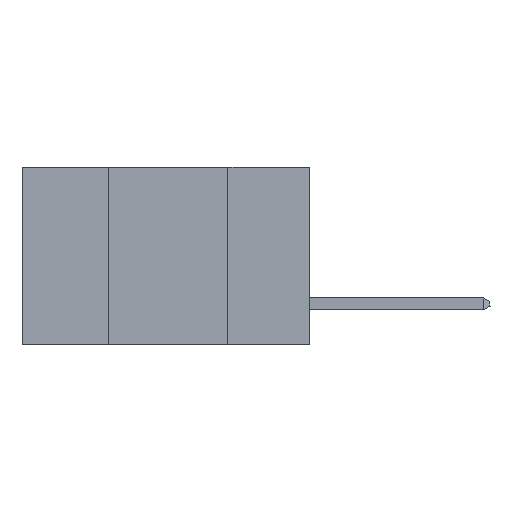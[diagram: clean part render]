
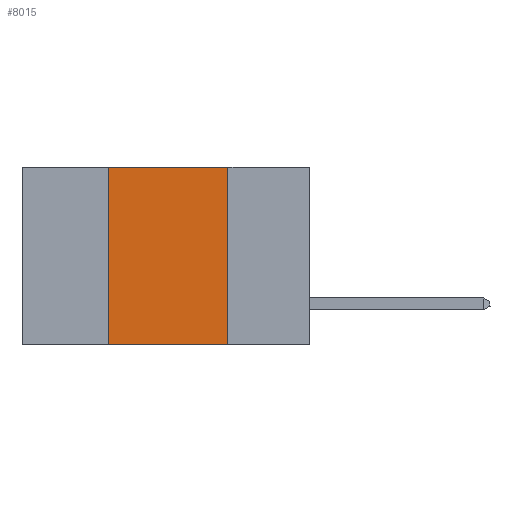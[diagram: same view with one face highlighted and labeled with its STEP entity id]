
A CAD part, left-side view. The second image highlights one B-rep face of the part: STEP entity #8015.
In plain terms, the highlighted planar face has unit normal (-1, 0, 0).
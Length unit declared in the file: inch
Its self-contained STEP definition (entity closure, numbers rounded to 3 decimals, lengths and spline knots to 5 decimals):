
#1480 = VERTEX_POINT ( 'NONE', #7869 ) ;
#1724 = ORIENTED_EDGE ( 'NONE', *, *, #2105, .F. ) ;
#2105 = EDGE_CURVE ( 'NONE', #18420, #6657, #20396, .T. ) ;
#2632 = VERTEX_POINT ( 'NONE', #9596 ) ;
#2825 = LINE ( 'NONE', #15860, #6782 ) ;
#4143 = EDGE_LOOP ( 'NONE', ( #13917, #4170, #1724, #4191 ) ) ;
#4170 = ORIENTED_EDGE ( 'NONE', *, *, #18962, .F. ) ;
#4191 = ORIENTED_EDGE ( 'NONE', *, *, #20231, .T. ) ;
#4377 = CARTESIAN_POINT ( 'NONE',  ( 0., 0.17, 0. ) ) ;
#4565 = VECTOR ( 'NONE', #16629, 39.37008 ) ;
#4564 = DIRECTION ( 'NONE',  ( 0., 0., -1. ) ) ;
#5582 = DIRECTION ( 'NONE',  ( 0., -1., 0. ) ) ;
#6474 = FACE_OUTER_BOUND ( 'NONE', #4143, .T. ) ;
#6653 = CARTESIAN_POINT ( 'NONE',  ( 0., 0.42, 0. ) ) ;
#6657 = VERTEX_POINT ( 'NONE', #16214 ) ;
#6782 = VECTOR ( 'NONE', #5582, 39.37008 ) ;
#7869 = CARTESIAN_POINT ( 'NONE',  ( 0., 0.17, 0. ) ) ;
#8015 = ADVANCED_FACE ( 'NONE', ( #6474 ), #12578, .F. ) ;
#9596 = CARTESIAN_POINT ( 'NONE',  ( 0., 0.17, -0.37 ) ) ;
#10068 = DIRECTION ( 'NONE',  ( 0., 0., -1. ) ) ;
#10157 = VECTOR ( 'NONE', #18342, 39.37008 ) ;
#10955 = CARTESIAN_POINT ( 'NONE',  ( 0., 0.6, 0. ) ) ;
#12189 = VECTOR ( 'NONE', #10068, 39.37008 ) ;
#12578 = PLANE ( 'NONE',  #15012 ) ;
#13059 = LINE ( 'NONE', #18613, #10157 ) ;
#13917 = ORIENTED_EDGE ( 'NONE', *, *, #21399, .F. ) ;
#14598 = LINE ( 'NONE', #4377, #12189 ) ;
#15012 = AXIS2_PLACEMENT_3D ( 'NONE', #10955, #15317, #4564 ) ;
#15317 = DIRECTION ( 'NONE',  ( 1., 0., 0. ) ) ;
#15860 = CARTESIAN_POINT ( 'NONE',  ( 0., 0.6, 0. ) ) ;
#16214 = CARTESIAN_POINT ( 'NONE',  ( 0., 0.42, 0. ) ) ;
#16629 = DIRECTION ( 'NONE',  ( 0., 0., 1. ) ) ;
#18342 = DIRECTION ( 'NONE',  ( 0., -1., 0. ) ) ;
#18420 = VERTEX_POINT ( 'NONE', #20919 ) ;
#18613 = CARTESIAN_POINT ( 'NONE',  ( 0., 0.6, -0.37 ) ) ;
#18962 = EDGE_CURVE ( 'NONE', #6657, #1480, #2825, .T. ) ;
#20231 = EDGE_CURVE ( 'NONE', #18420, #2632, #13059, .T. ) ;
#20396 = LINE ( 'NONE', #6653, #4565 ) ;
#20919 = CARTESIAN_POINT ( 'NONE',  ( 0., 0.42, -0.37 ) ) ;
#21399 = EDGE_CURVE ( 'NONE', #1480, #2632, #14598, .T. ) ;
